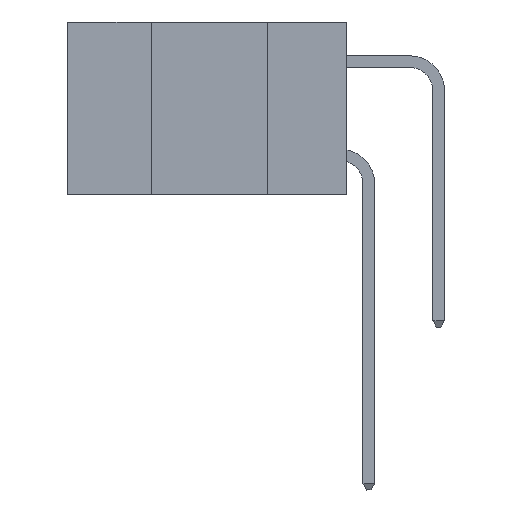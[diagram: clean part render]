
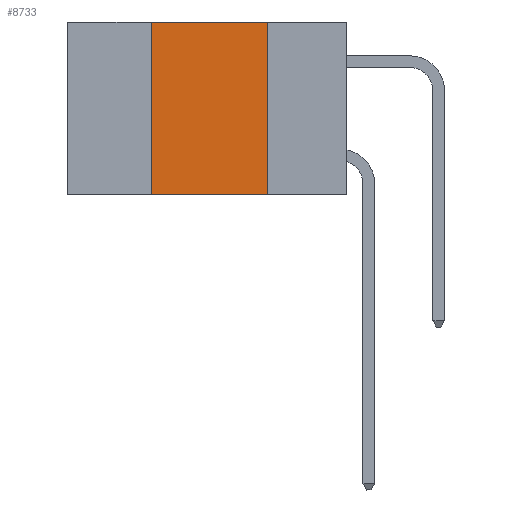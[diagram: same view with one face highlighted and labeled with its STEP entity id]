
A CAD part, left-side view. The second image highlights one B-rep face of the part: STEP entity #8733.
In plain terms, the highlighted planar face has unit normal (-1, 0, 0).
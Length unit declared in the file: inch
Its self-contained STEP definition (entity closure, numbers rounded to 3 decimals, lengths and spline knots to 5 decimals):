
#1574 = LINE ( 'NONE', #29015, #3477 ) ;
#1903 = DIRECTION ( 'NONE',  ( 0., 0., -1. ) ) ;
#2442 = VERTEX_POINT ( 'NONE', #17562 ) ;
#3477 = VECTOR ( 'NONE', #4491, 39.37008 ) ;
#4491 = DIRECTION ( 'NONE',  ( 0., 0., 1. ) ) ;
#4641 = EDGE_LOOP ( 'NONE', ( #15265, #24279, #9355, #20166 ) ) ;
#4751 = CARTESIAN_POINT ( 'NONE',  ( 0., 0.6, 0. ) ) ;
#4803 = LINE ( 'NONE', #25270, #15823 ) ;
#5112 = VERTEX_POINT ( 'NONE', #29873 ) ;
#5826 = VECTOR ( 'NONE', #19087, 39.37008 ) ;
#6214 = FACE_OUTER_BOUND ( 'NONE', #4641, .T. ) ;
#7538 = VERTEX_POINT ( 'NONE', #28229 ) ;
#8733 = ADVANCED_FACE ( 'NONE', ( #6214 ), #21740, .F. ) ;
#9355 = ORIENTED_EDGE ( 'NONE', *, *, #25967, .F. ) ;
#11601 = CARTESIAN_POINT ( 'NONE',  ( 0., 0.17, 0. ) ) ;
#12032 = DIRECTION ( 'NONE',  ( 1., 0., 0. ) ) ;
#12490 = EDGE_CURVE ( 'NONE', #2442, #7538, #4803, .T. ) ;
#14019 = EDGE_CURVE ( 'NONE', #31361, #5112, #18743, .T. ) ;
#15265 = ORIENTED_EDGE ( 'NONE', *, *, #20846, .F. ) ;
#15823 = VECTOR ( 'NONE', #15876, 39.37008 ) ;
#15876 = DIRECTION ( 'NONE',  ( 0., -1., 0. ) ) ;
#17562 = CARTESIAN_POINT ( 'NONE',  ( 0., 0.42, -0.37 ) ) ;
#18743 = LINE ( 'NONE', #18889, #5826 ) ;
#18889 = CARTESIAN_POINT ( 'NONE',  ( 0., 0.6, 0. ) ) ;
#19087 = DIRECTION ( 'NONE',  ( 0., -1., 0. ) ) ;
#20166 = ORIENTED_EDGE ( 'NONE', *, *, #12490, .T. ) ;
#20846 = EDGE_CURVE ( 'NONE', #5112, #7538, #26057, .T. ) ;
#21740 = PLANE ( 'NONE',  #25860 ) ;
#23767 = VECTOR ( 'NONE', #1903, 39.37008 ) ;
#24279 = ORIENTED_EDGE ( 'NONE', *, *, #14019, .F. ) ;
#25270 = CARTESIAN_POINT ( 'NONE',  ( 0., 0.6, -0.37 ) ) ;
#25860 = AXIS2_PLACEMENT_3D ( 'NONE', #4751, #12032, #28963 ) ;
#25967 = EDGE_CURVE ( 'NONE', #2442, #31361, #1574, .T. ) ;
#26057 = LINE ( 'NONE', #11601, #23767 ) ;
#26544 = CARTESIAN_POINT ( 'NONE',  ( 0., 0.42, 0. ) ) ;
#28229 = CARTESIAN_POINT ( 'NONE',  ( 0., 0.17, -0.37 ) ) ;
#28963 = DIRECTION ( 'NONE',  ( 0., 0., -1. ) ) ;
#29015 = CARTESIAN_POINT ( 'NONE',  ( 0., 0.42, 0. ) ) ;
#29873 = CARTESIAN_POINT ( 'NONE',  ( 0., 0.17, 0. ) ) ;
#31361 = VERTEX_POINT ( 'NONE', #26544 ) ;
